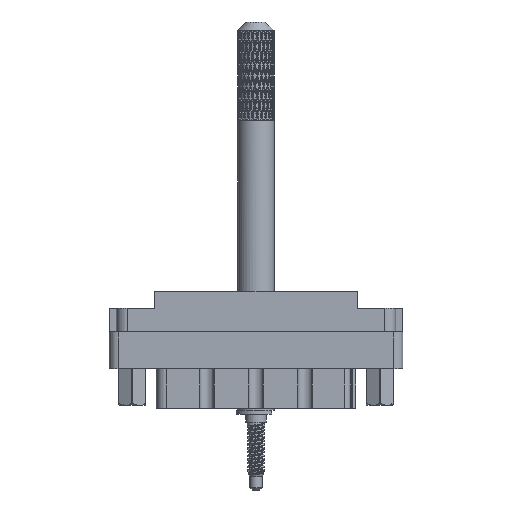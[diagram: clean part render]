
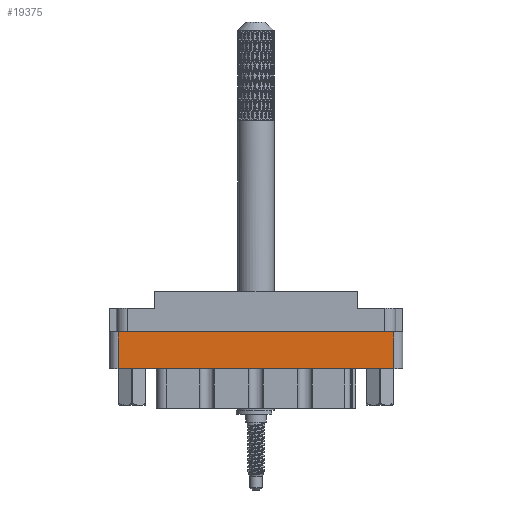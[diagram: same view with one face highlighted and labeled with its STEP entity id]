
A CAD part, front view. The second image highlights one B-rep face of the part: STEP entity #19375.
In plain terms, the highlighted planar face has unit normal (0, -1, 0).
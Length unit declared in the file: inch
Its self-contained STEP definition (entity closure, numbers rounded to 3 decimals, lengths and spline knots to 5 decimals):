
#5442 = CARTESIAN_POINT ( 'NONE',  ( 0.938, -0.438, -0.277 ) ) ;
#5587 = VECTOR ( 'NONE', #103107, 39.37008 ) ;
#9641 = EDGE_CURVE ( 'NONE', #40510, #38447, #10439, .T. ) ;
#10439 = LINE ( 'NONE', #108203, #108185 ) ;
#11714 = ORIENTED_EDGE ( 'NONE', *, *, #67782, .F. ) ;
#12304 = DIRECTION ( 'NONE',  ( 0., -1., 0. ) ) ;
#15920 = CARTESIAN_POINT ( 'NONE',  ( -0.938, -0.438, -0.529 ) ) ;
#17055 = EDGE_CURVE ( 'NONE', #40510, #56345, #82189, .T. ) ;
#19375 = ADVANCED_FACE ( 'NONE', ( #50274 ), #53766, .T. ) ;
#20820 = DIRECTION ( 'NONE',  ( 0., 0., -1. ) ) ;
#26936 = ORIENTED_EDGE ( 'NONE', *, *, #68869, .T. ) ;
#28834 = CARTESIAN_POINT ( 'NONE',  ( 0.938, -0.438, -0.529 ) ) ;
#37413 = DIRECTION ( 'NONE',  ( 1., 0., 0. ) ) ;
#38363 = VECTOR ( 'NONE', #37413, 39.37008 ) ;
#38447 = VERTEX_POINT ( 'NONE', #5442 ) ;
#40510 = VERTEX_POINT ( 'NONE', #28834 ) ;
#50274 = FACE_OUTER_BOUND ( 'NONE', #74428, .T. ) ;
#53372 = CARTESIAN_POINT ( 'NONE',  ( 0., -0.438, -0.529 ) ) ;
#53766 = PLANE ( 'NONE',  #88824 ) ;
#56345 = VERTEX_POINT ( 'NONE', #15920 ) ;
#56662 = VECTOR ( 'NONE', #88342, 39.37008 ) ;
#57710 = DIRECTION ( 'NONE',  ( 0., 0., 1. ) ) ;
#63563 = CARTESIAN_POINT ( 'NONE',  ( 0., -0.438, -0.277 ) ) ;
#65799 = ORIENTED_EDGE ( 'NONE', *, *, #17055, .F. ) ;
#67782 = EDGE_CURVE ( 'NONE', #83609, #38447, #83155, .T. ) ;
#68869 = EDGE_CURVE ( 'NONE', #83609, #56345, #106766, .T. ) ;
#70149 = CARTESIAN_POINT ( 'NONE',  ( -0.938, -0.438, -0.277 ) ) ;
#70658 = CARTESIAN_POINT ( 'NONE',  ( -1., -0.438, -0.798 ) ) ;
#74428 = EDGE_LOOP ( 'NONE', ( #11714, #26936, #65799, #85378 ) ) ;
#82189 = LINE ( 'NONE', #53372, #5587 ) ;
#83155 = LINE ( 'NONE', #63563, #38363 ) ;
#83609 = VERTEX_POINT ( 'NONE', #70149 ) ;
#85378 = ORIENTED_EDGE ( 'NONE', *, *, #9641, .T. ) ;
#88342 = DIRECTION ( 'NONE',  ( 0., 0., -1. ) ) ;
#88824 = AXIS2_PLACEMENT_3D ( 'NONE', #70658, #12304, #20820 ) ;
#89461 = CARTESIAN_POINT ( 'NONE',  ( -0.938, -0.438, -0.798 ) ) ;
#103107 = DIRECTION ( 'NONE',  ( -1., 0., 0. ) ) ;
#106766 = LINE ( 'NONE', #89461, #56662 ) ;
#108185 = VECTOR ( 'NONE', #57710, 39.37008 ) ;
#108203 = CARTESIAN_POINT ( 'NONE',  ( 0.938, -0.438, -0.798 ) ) ;
